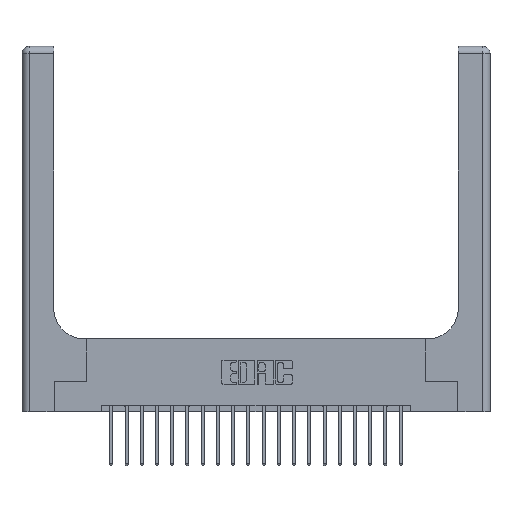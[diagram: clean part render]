
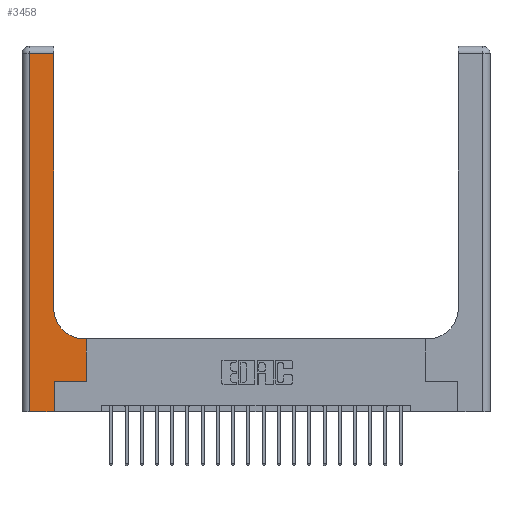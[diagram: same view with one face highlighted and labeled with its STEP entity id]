
A CAD part, top view. The second image highlights one B-rep face of the part: STEP entity #3458.
In plain terms, the highlighted planar face has unit normal (0, 0, 1).
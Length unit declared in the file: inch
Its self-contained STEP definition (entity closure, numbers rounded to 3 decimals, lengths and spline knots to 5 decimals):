
#240 = CARTESIAN_POINT ( 'NONE',  ( 0.265, 0., 0.37 ) ) ;
#637 = VERTEX_POINT ( 'NONE', #2923 ) ;
#1192 = LINE ( 'NONE', #13454, #18101 ) ;
#1475 = ORIENTED_EDGE ( 'NONE', *, *, #20293, .T. ) ;
#1530 = VERTEX_POINT ( 'NONE', #3260 ) ;
#1532 = CARTESIAN_POINT ( 'NONE',  ( 0., 0., 0.37 ) ) ;
#1561 = CARTESIAN_POINT ( 'NONE',  ( 0.528, 0.25, 0.37 ) ) ;
#1854 = ORIENTED_EDGE ( 'NONE', *, *, #15342, .T. ) ;
#2077 = DIRECTION ( 'NONE',  ( 0., 1., 0. ) ) ;
#2670 = PLANE ( 'NONE',  #3843 ) ;
#2698 = ORIENTED_EDGE ( 'NONE', *, *, #10230, .T. ) ;
#2923 = CARTESIAN_POINT ( 'NONE',  ( 0.06, 0., 0.37 ) ) ;
#3177 = ORIENTED_EDGE ( 'NONE', *, *, #8143, .T. ) ;
#3260 = CARTESIAN_POINT ( 'NONE',  ( 0.51, 0.6, 0.37 ) ) ;
#3458 = ADVANCED_FACE ( 'NONE', ( #20872 ), #2670, .F. ) ;
#3525 = DIRECTION ( 'NONE',  ( 0., 1., 0. ) ) ;
#3843 = AXIS2_PLACEMENT_3D ( 'NONE', #4240, #19152, #14104 ) ;
#3926 = VECTOR ( 'NONE', #2077, 39.37008 ) ;
#3942 = LINE ( 'NONE', #13881, #10091 ) ;
#4240 = CARTESIAN_POINT ( 'NONE',  ( 0., 3., 0.37 ) ) ;
#4320 = VERTEX_POINT ( 'NONE', #12976 ) ;
#4411 = CARTESIAN_POINT ( 'NONE',  ( 0.265, 0.25, 0.37 ) ) ;
#4696 = CARTESIAN_POINT ( 'NONE',  ( 0., 2.94, 0.37 ) ) ;
#4859 = EDGE_CURVE ( 'NONE', #4320, #9319, #8470, .T. ) ;
#5751 = AXIS2_PLACEMENT_3D ( 'NONE', #14287, #9357, #6123 ) ;
#5904 = CARTESIAN_POINT ( 'NONE',  ( 0.06, 2.94, 0.37 ) ) ;
#6123 = DIRECTION ( 'NONE',  ( 1., 0., 0. ) ) ;
#6498 = LINE ( 'NONE', #7199, #3926 ) ;
#6712 = DIRECTION ( 'NONE',  ( 1., 0., 0. ) ) ;
#6792 = CARTESIAN_POINT ( 'NONE',  ( 0.528, 0.25, 0.37 ) ) ;
#7199 = CARTESIAN_POINT ( 'NONE',  ( 0.26, 3., 0.37 ) ) ;
#7461 = CARTESIAN_POINT ( 'NONE',  ( 0.528, 0.6, 0.37 ) ) ;
#7856 = ORIENTED_EDGE ( 'NONE', *, *, #10967, .T. ) ;
#8143 = EDGE_CURVE ( 'NONE', #637, #4320, #11212, .T. ) ;
#8226 = DIRECTION ( 'NONE',  ( 0., 1., 0. ) ) ;
#8470 = LINE ( 'NONE', #240, #9236 ) ;
#8649 = CARTESIAN_POINT ( 'NONE',  ( 0.26, 0.85, 0.37 ) ) ;
#9236 = VECTOR ( 'NONE', #3525, 39.37008 ) ;
#9319 = VERTEX_POINT ( 'NONE', #4411 ) ;
#9357 = DIRECTION ( 'NONE',  ( 0., 0., -1. ) ) ;
#9473 = DIRECTION ( 'NONE',  ( 1., 0., 0. ) ) ;
#9929 = VECTOR ( 'NONE', #9473, 39.37008 ) ;
#10044 = CARTESIAN_POINT ( 'NONE',  ( 0.06, 3., 0.37 ) ) ;
#10091 = VECTOR ( 'NONE', #15527, 39.37008 ) ;
#10230 = EDGE_CURVE ( 'NONE', #15916, #1530, #3942, .T. ) ;
#10967 = EDGE_CURVE ( 'NONE', #20642, #12806, #15684, .T. ) ;
#11168 = VECTOR ( 'NONE', #14839, 39.37008 ) ;
#11212 = LINE ( 'NONE', #1532, #9929 ) ;
#11444 = EDGE_CURVE ( 'NONE', #12087, #20642, #6498, .T. ) ;
#11785 = ORIENTED_EDGE ( 'NONE', *, *, #20826, .T. ) ;
#12087 = VERTEX_POINT ( 'NONE', #8649 ) ;
#12112 = LINE ( 'NONE', #6792, #18562 ) ;
#12710 = DIRECTION ( 'NONE',  ( -1., 0., 0. ) ) ;
#12806 = VERTEX_POINT ( 'NONE', #5904 ) ;
#12976 = CARTESIAN_POINT ( 'NONE',  ( 0.265, 0., 0.37 ) ) ;
#13239 = LINE ( 'NONE', #10044, #11168 ) ;
#13454 = CARTESIAN_POINT ( 'NONE',  ( 0.265, 0.25, 0.37 ) ) ;
#13881 = CARTESIAN_POINT ( 'NONE',  ( 0.26, 0.6, 0.37 ) ) ;
#14104 = DIRECTION ( 'NONE',  ( -1., 0., 0. ) ) ;
#14234 = VERTEX_POINT ( 'NONE', #1561 ) ;
#14287 = CARTESIAN_POINT ( 'NONE',  ( 0.51, 0.85, 0.37 ) ) ;
#14839 = DIRECTION ( 'NONE',  ( 0., -1., 0. ) ) ;
#14909 = EDGE_CURVE ( 'NONE', #14234, #15916, #12112, .T. ) ;
#15342 = EDGE_CURVE ( 'NONE', #1530, #12087, #19837, .T. ) ;
#15527 = DIRECTION ( 'NONE',  ( -1., 0., 0. ) ) ;
#15684 = LINE ( 'NONE', #4696, #18818 ) ;
#15916 = VERTEX_POINT ( 'NONE', #7461 ) ;
#15974 = ORIENTED_EDGE ( 'NONE', *, *, #14909, .T. ) ;
#16223 = CARTESIAN_POINT ( 'NONE',  ( 0.26, 2.94, 0.37 ) ) ;
#16889 = EDGE_LOOP ( 'NONE', ( #18918, #7856, #1475, #3177, #20983, #11785, #15974, #2698, #1854 ) ) ;
#18101 = VECTOR ( 'NONE', #6712, 39.37008 ) ;
#18562 = VECTOR ( 'NONE', #8226, 39.37008 ) ;
#18818 = VECTOR ( 'NONE', #12710, 39.37008 ) ;
#18918 = ORIENTED_EDGE ( 'NONE', *, *, #11444, .T. ) ;
#19152 = DIRECTION ( 'NONE',  ( 0., 0., -1. ) ) ;
#19837 = CIRCLE ( 'NONE', #5751, 0.25 ) ;
#20293 = EDGE_CURVE ( 'NONE', #12806, #637, #13239, .T. ) ;
#20642 = VERTEX_POINT ( 'NONE', #16223 ) ;
#20826 = EDGE_CURVE ( 'NONE', #9319, #14234, #1192, .T. ) ;
#20872 = FACE_OUTER_BOUND ( 'NONE', #16889, .T. ) ;
#20983 = ORIENTED_EDGE ( 'NONE', *, *, #4859, .T. ) ;
